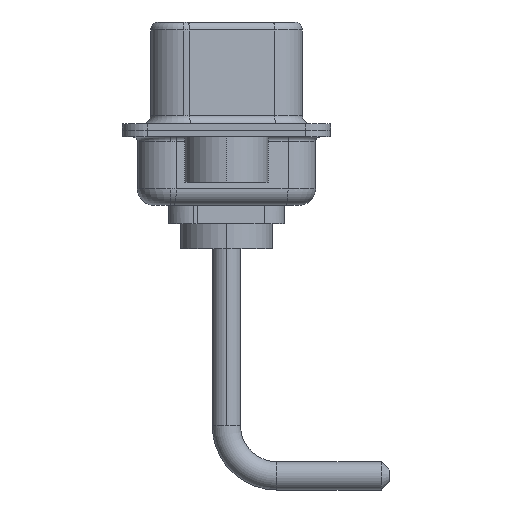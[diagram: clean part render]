
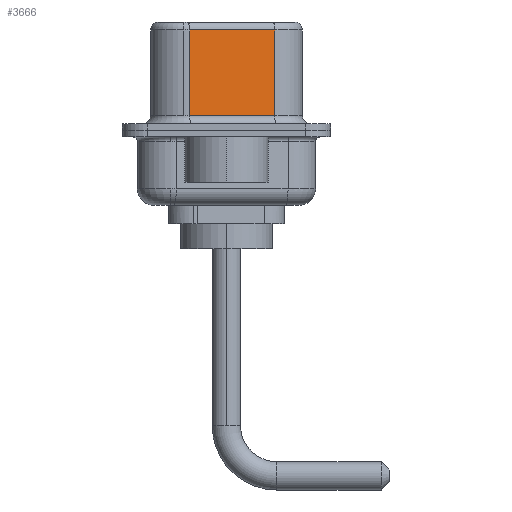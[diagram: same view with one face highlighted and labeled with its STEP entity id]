
A CAD part, left-side view. The second image highlights one B-rep face of the part: STEP entity #3666.
In plain terms, the highlighted planar face has unit normal (-0.985, -0.174, 0).
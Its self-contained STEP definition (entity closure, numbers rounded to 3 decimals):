
#652 = VECTOR ( 'NONE', #11093, 1000. ) ;
#1053 = CARTESIAN_POINT ( 'NONE',  ( 4.58, -2.897, 0.9 ) ) ;
#1279 = EDGE_LOOP ( 'NONE', ( #7048, #3644, #4332, #11314 ) ) ;
#1512 = EDGE_CURVE ( 'NONE', #12334, #2919, #12790, .T. ) ;
#2919 = VERTEX_POINT ( 'NONE', #1053 ) ;
#2962 = PLANE ( 'NONE',  #4652 ) ;
#3118 = DIRECTION ( 'NONE',  ( -0.174, 0.985, 0. ) ) ;
#3644 = ORIENTED_EDGE ( 'NONE', *, *, #12261, .T. ) ;
#3666 = ADVANCED_FACE ( 'NONE', ( #13245 ), #2962, .F. ) ;
#4038 = CARTESIAN_POINT ( 'NONE',  ( 3.68, 2.203, 0.9 ) ) ;
#4208 = VECTOR ( 'NONE', #8797, 1000. ) ;
#4332 = ORIENTED_EDGE ( 'NONE', *, *, #11961, .T. ) ;
#4652 = AXIS2_PLACEMENT_3D ( 'NONE', #6695, #12022, #3118 ) ;
#4870 = LINE ( 'NONE', #7400, #4208 ) ;
#5500 = VECTOR ( 'NONE', #14211, 1000. ) ;
#5613 = CARTESIAN_POINT ( 'NONE',  ( 3.68, 2.203, 6.52 ) ) ;
#6695 = CARTESIAN_POINT ( 'NONE',  ( 4.58, -2.897, 6.52 ) ) ;
#7048 = ORIENTED_EDGE ( 'NONE', *, *, #1512, .F. ) ;
#7400 = CARTESIAN_POINT ( 'NONE',  ( 4.58, -2.897, 6.02 ) ) ;
#8261 = VECTOR ( 'NONE', #10166, 1000. ) ;
#8638 = EDGE_CURVE ( 'NONE', #9426, #2919, #14596, .T. ) ;
#8797 = DIRECTION ( 'NONE',  ( -0.174, 0.985, 0. ) ) ;
#9099 = CARTESIAN_POINT ( 'NONE',  ( 4.58, -2.897, 6.52 ) ) ;
#9426 = VERTEX_POINT ( 'NONE', #4038 ) ;
#9785 = CARTESIAN_POINT ( 'NONE',  ( 4.58, -2.897, 6.02 ) ) ;
#10166 = DIRECTION ( 'NONE',  ( 0., 0., -1. ) ) ;
#10290 = LINE ( 'NONE', #5613, #5500 ) ;
#10916 = VERTEX_POINT ( 'NONE', #13417 ) ;
#11093 = DIRECTION ( 'NONE',  ( 0.174, -0.985, 0. ) ) ;
#11314 = ORIENTED_EDGE ( 'NONE', *, *, #8638, .T. ) ;
#11961 = EDGE_CURVE ( 'NONE', #10916, #9426, #10290, .T. ) ;
#12022 = DIRECTION ( 'NONE',  ( 0.985, 0.174, 0. ) ) ;
#12261 = EDGE_CURVE ( 'NONE', #12334, #10916, #4870, .T. ) ;
#12334 = VERTEX_POINT ( 'NONE', #9785 ) ;
#12790 = LINE ( 'NONE', #9099, #8261 ) ;
#13245 = FACE_OUTER_BOUND ( 'NONE', #1279, .T. ) ;
#13417 = CARTESIAN_POINT ( 'NONE',  ( 3.68, 2.203, 6.02 ) ) ;
#13536 = CARTESIAN_POINT ( 'NONE',  ( 4.58, -2.897, 0.9 ) ) ;
#14211 = DIRECTION ( 'NONE',  ( 0., 0., -1. ) ) ;
#14596 = LINE ( 'NONE', #13536, #652 ) ;
